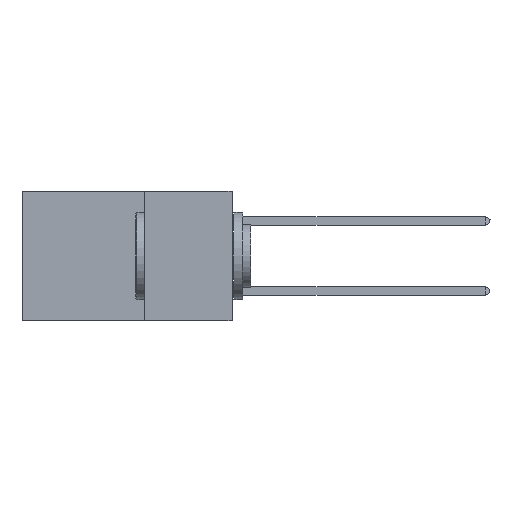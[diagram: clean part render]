
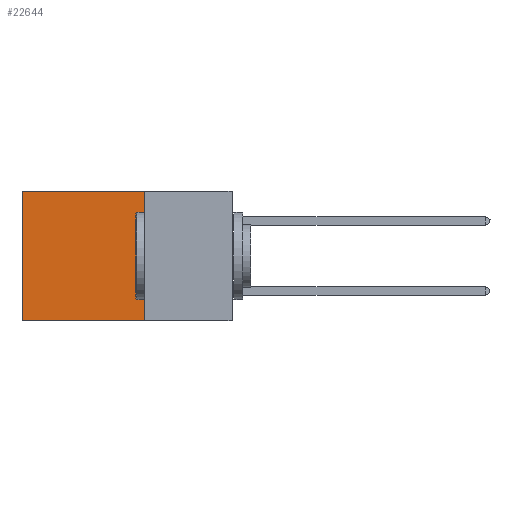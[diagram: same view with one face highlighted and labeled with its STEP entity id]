
A CAD part, left-side view. The second image highlights one B-rep face of the part: STEP entity #22644.
In plain terms, the highlighted planar face has unit normal (-1, 0, 0).
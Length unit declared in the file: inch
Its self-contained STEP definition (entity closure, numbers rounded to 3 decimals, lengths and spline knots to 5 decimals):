
#50 = EDGE_CURVE ( 'NONE', #1241, #16869, #5397, .T. ) ;
#257 = AXIS2_PLACEMENT_3D ( 'NONE', #15449, #2571, #17576 ) ;
#1241 = VERTEX_POINT ( 'NONE', #4414 ) ;
#2571 = DIRECTION ( 'NONE',  ( 1., 0., 0. ) ) ;
#4078 = EDGE_CURVE ( 'NONE', #17190, #8077, #24588, .T. ) ;
#4414 = CARTESIAN_POINT ( 'NONE',  ( 0.2875, 0.25, 0. ) ) ;
#4490 = LINE ( 'NONE', #4918, #10914 ) ;
#4918 = CARTESIAN_POINT ( 'NONE',  ( 0.2875, 0.25, -0.37 ) ) ;
#5397 = LINE ( 'NONE', #13141, #16491 ) ;
#5823 = EDGE_CURVE ( 'NONE', #16869, #8077, #4490, .T. ) ;
#6153 = DIRECTION ( 'NONE',  ( 0., 0., -1. ) ) ;
#6201 = VECTOR ( 'NONE', #6408, 39.37008 ) ;
#6408 = DIRECTION ( 'NONE',  ( 0., 1., 0. ) ) ;
#6875 = LINE ( 'NONE', #10666, #6201 ) ;
#7220 = CARTESIAN_POINT ( 'NONE',  ( 0.2875, 0.25, -0.37 ) ) ;
#7469 = DIRECTION ( 'NONE',  ( 0., 0., -1. ) ) ;
#7498 = CARTESIAN_POINT ( 'NONE',  ( 0.2875, 0.6, -0.37 ) ) ;
#8077 = VERTEX_POINT ( 'NONE', #7498 ) ;
#10666 = CARTESIAN_POINT ( 'NONE',  ( 0.2875, 0.25, 0. ) ) ;
#10872 = ORIENTED_EDGE ( 'NONE', *, *, #4078, .T. ) ;
#10914 = VECTOR ( 'NONE', #11337, 39.37008 ) ;
#11337 = DIRECTION ( 'NONE',  ( 0., 1., 0. ) ) ;
#12558 = CARTESIAN_POINT ( 'NONE',  ( 0.2875, 0.6, 0. ) ) ;
#13141 = CARTESIAN_POINT ( 'NONE',  ( 0.2875, 0.25, 0. ) ) ;
#15449 = CARTESIAN_POINT ( 'NONE',  ( 0.2875, 0.25, 0. ) ) ;
#16491 = VECTOR ( 'NONE', #6153, 39.37008 ) ;
#16869 = VERTEX_POINT ( 'NONE', #7220 ) ;
#16952 = EDGE_LOOP ( 'NONE', ( #10872, #23517, #25500, #21660 ) ) ;
#17190 = VERTEX_POINT ( 'NONE', #12558 ) ;
#17576 = DIRECTION ( 'NONE',  ( 0., 0., -1. ) ) ;
#17589 = VECTOR ( 'NONE', #7469, 39.37008 ) ;
#17939 = EDGE_CURVE ( 'NONE', #1241, #17190, #6875, .T. ) ;
#18075 = CARTESIAN_POINT ( 'NONE',  ( 0.2875, 0.6, 0. ) ) ;
#21660 = ORIENTED_EDGE ( 'NONE', *, *, #17939, .T. ) ;
#21751 = PLANE ( 'NONE',  #257 ) ;
#22644 = ADVANCED_FACE ( 'NONE', ( #27769 ), #21751, .F. ) ;
#23517 = ORIENTED_EDGE ( 'NONE', *, *, #5823, .F. ) ;
#24588 = LINE ( 'NONE', #18075, #17589 ) ;
#25500 = ORIENTED_EDGE ( 'NONE', *, *, #50, .F. ) ;
#27769 = FACE_OUTER_BOUND ( 'NONE', #16952, .T. ) ;
